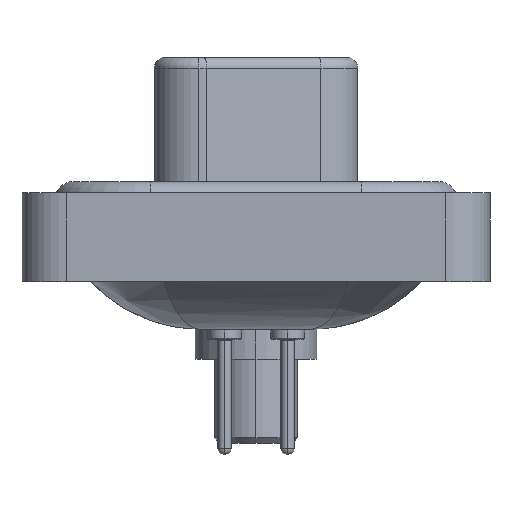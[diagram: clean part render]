
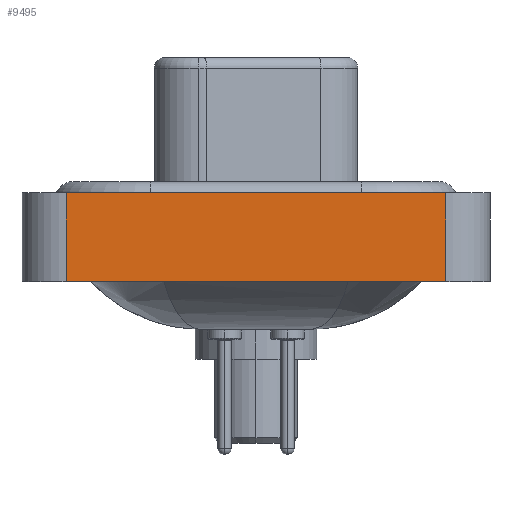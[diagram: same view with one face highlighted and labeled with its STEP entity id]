
A CAD part, left-side view. The second image highlights one B-rep face of the part: STEP entity #9495.
In plain terms, the highlighted planar face has unit normal (-1, 0, 0).
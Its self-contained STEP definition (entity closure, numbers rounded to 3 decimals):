
#299 = CARTESIAN_POINT ( 'NONE',  ( -7.3, -8.55, -3.6 ) ) ;
#500 = CARTESIAN_POINT ( 'NONE',  ( -7.3, 8.55, -3.6 ) ) ;
#768 = EDGE_LOOP ( 'NONE', ( #6570, #18533, #16790, #2218 ) ) ;
#1481 = CARTESIAN_POINT ( 'NONE',  ( -7.3, -8.55, 0.4 ) ) ;
#2218 = ORIENTED_EDGE ( 'NONE', *, *, #13296, .T. ) ;
#3225 = CARTESIAN_POINT ( 'NONE',  ( -7.3, -8.55, -3.6 ) ) ;
#3284 = CARTESIAN_POINT ( 'NONE',  ( -7.3, -8.55, -3.6 ) ) ;
#3709 = DIRECTION ( 'NONE',  ( 0., 0., 1. ) ) ;
#3986 = DIRECTION ( 'NONE',  ( 0., -1., 0. ) ) ;
#4244 = VERTEX_POINT ( 'NONE', #3284 ) ;
#4495 = DIRECTION ( 'NONE',  ( 0., -1., 0. ) ) ;
#5186 = LINE ( 'NONE', #500, #15077 ) ;
#6570 = ORIENTED_EDGE ( 'NONE', *, *, #13510, .T. ) ;
#7793 = EDGE_CURVE ( 'NONE', #12660, #8880, #5186, .T. ) ;
#8880 = VERTEX_POINT ( 'NONE', #20150 ) ;
#9495 = ADVANCED_FACE ( 'NONE', ( #13208 ), #9718, .T. ) ;
#9718 = PLANE ( 'NONE',  #9963 ) ;
#9963 = AXIS2_PLACEMENT_3D ( 'NONE', #299, #11421, #3709 ) ;
#10740 = LINE ( 'NONE', #3225, #11192 ) ;
#11192 = VECTOR ( 'NONE', #12838, 1000. ) ;
#11421 = DIRECTION ( 'NONE',  ( -1., 0., 0. ) ) ;
#11630 = DIRECTION ( 'NONE',  ( 0., 0., 1. ) ) ;
#12525 = LINE ( 'NONE', #12622, #16915 ) ;
#12622 = CARTESIAN_POINT ( 'NONE',  ( -7.3, -8.55, 0.4 ) ) ;
#12660 = VERTEX_POINT ( 'NONE', #19937 ) ;
#12838 = DIRECTION ( 'NONE',  ( 0., 0., 1. ) ) ;
#13208 = FACE_OUTER_BOUND ( 'NONE', #768, .T. ) ;
#13296 = EDGE_CURVE ( 'NONE', #12660, #4244, #18495, .T. ) ;
#13390 = CARTESIAN_POINT ( 'NONE',  ( -7.3, -8.55, -3.6 ) ) ;
#13510 = EDGE_CURVE ( 'NONE', #4244, #18510, #10740, .T. ) ;
#15077 = VECTOR ( 'NONE', #11630, 1000. ) ;
#16782 = EDGE_CURVE ( 'NONE', #8880, #18510, #12525, .T. ) ;
#16790 = ORIENTED_EDGE ( 'NONE', *, *, #7793, .F. ) ;
#16915 = VECTOR ( 'NONE', #4495, 1000. ) ;
#18282 = VECTOR ( 'NONE', #3986, 1000. ) ;
#18495 = LINE ( 'NONE', #13390, #18282 ) ;
#18510 = VERTEX_POINT ( 'NONE', #1481 ) ;
#18533 = ORIENTED_EDGE ( 'NONE', *, *, #16782, .F. ) ;
#19937 = CARTESIAN_POINT ( 'NONE',  ( -7.3, 8.55, -3.6 ) ) ;
#20150 = CARTESIAN_POINT ( 'NONE',  ( -7.3, 8.55, 0.4 ) ) ;
